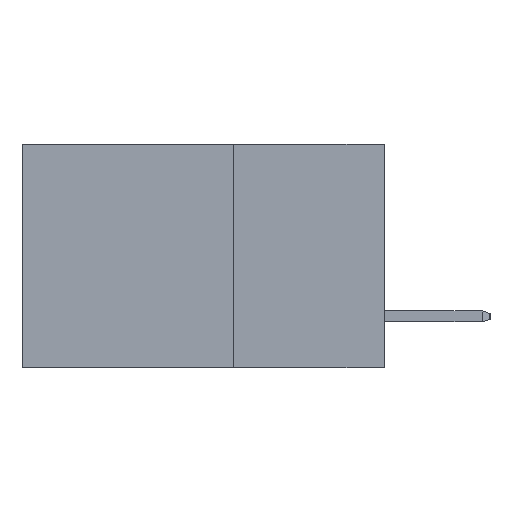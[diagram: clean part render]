
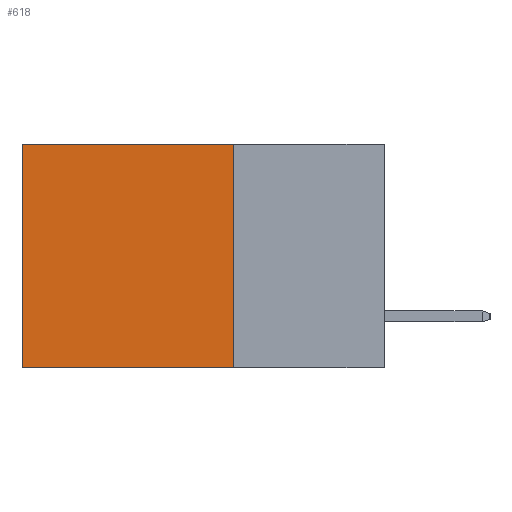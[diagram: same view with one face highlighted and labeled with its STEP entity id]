
A CAD part, left-side view. The second image highlights one B-rep face of the part: STEP entity #618.
In plain terms, the highlighted planar face has unit normal (-1, 0, 0).
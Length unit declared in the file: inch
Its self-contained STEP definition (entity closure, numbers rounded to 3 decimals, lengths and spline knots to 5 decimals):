
#109 = DIRECTION ( 'NONE',  ( 0., 0., -1. ) ) ;
#618 = ADVANCED_FACE ( 'NONE', ( #10779 ), #743, .F. ) ;
#743 = PLANE ( 'NONE',  #5560 ) ;
#899 = CARTESIAN_POINT ( 'NONE',  ( 0.2615, 0.25, -0.37 ) ) ;
#1094 = CARTESIAN_POINT ( 'NONE',  ( 0.2615, 0.6, 0. ) ) ;
#1648 = EDGE_CURVE ( 'NONE', #4680, #8772, #9428, .T. ) ;
#2217 = VECTOR ( 'NONE', #109, 39.37008 ) ;
#2409 = ORIENTED_EDGE ( 'NONE', *, *, #6695, .F. ) ;
#3757 = CARTESIAN_POINT ( 'NONE',  ( 0.2615, 0.25, 0. ) ) ;
#3794 = EDGE_LOOP ( 'NONE', ( #9973, #12274, #2409, #10246 ) ) ;
#4482 = DIRECTION ( 'NONE',  ( 0., 1., 0. ) ) ;
#4680 = VERTEX_POINT ( 'NONE', #7000 ) ;
#4909 = CARTESIAN_POINT ( 'NONE',  ( 0.2615, 0.25, 0. ) ) ;
#5096 = LINE ( 'NONE', #4909, #7651 ) ;
#5403 = DIRECTION ( 'NONE',  ( 0., 0., -1. ) ) ;
#5560 = AXIS2_PLACEMENT_3D ( 'NONE', #5653, #7564, #7445 ) ;
#5578 = CARTESIAN_POINT ( 'NONE',  ( 0.2615, 0.25, -0.37 ) ) ;
#5653 = CARTESIAN_POINT ( 'NONE',  ( 0.2615, 0.25, -0.37 ) ) ;
#5896 = VECTOR ( 'NONE', #5403, 39.37008 ) ;
#6272 = CARTESIAN_POINT ( 'NONE',  ( 0.2615, 0.6, -0.37 ) ) ;
#6695 = EDGE_CURVE ( 'NONE', #12496, #4680, #8741, .T. ) ;
#7000 = CARTESIAN_POINT ( 'NONE',  ( 0.2615, 0.25, -0.37 ) ) ;
#7445 = DIRECTION ( 'NONE',  ( 0., 0., -1. ) ) ;
#7564 = DIRECTION ( 'NONE',  ( 1., 0., 0. ) ) ;
#7651 = VECTOR ( 'NONE', #10583, 39.37008 ) ;
#8472 = CARTESIAN_POINT ( 'NONE',  ( 0.2615, 0.6, -0.37 ) ) ;
#8533 = EDGE_CURVE ( 'NONE', #12496, #8834, #5096, .T. ) ;
#8741 = LINE ( 'NONE', #5578, #5896 ) ;
#8772 = VERTEX_POINT ( 'NONE', #6272 ) ;
#8834 = VERTEX_POINT ( 'NONE', #1094 ) ;
#8863 = VECTOR ( 'NONE', #4482, 39.37008 ) ;
#9428 = LINE ( 'NONE', #899, #8863 ) ;
#9973 = ORIENTED_EDGE ( 'NONE', *, *, #10653, .T. ) ;
#10108 = LINE ( 'NONE', #8472, #2217 ) ;
#10246 = ORIENTED_EDGE ( 'NONE', *, *, #8533, .T. ) ;
#10583 = DIRECTION ( 'NONE',  ( 0., 1., 0. ) ) ;
#10653 = EDGE_CURVE ( 'NONE', #8834, #8772, #10108, .T. ) ;
#10779 = FACE_OUTER_BOUND ( 'NONE', #3794, .T. ) ;
#12274 = ORIENTED_EDGE ( 'NONE', *, *, #1648, .F. ) ;
#12496 = VERTEX_POINT ( 'NONE', #3757 ) ;
